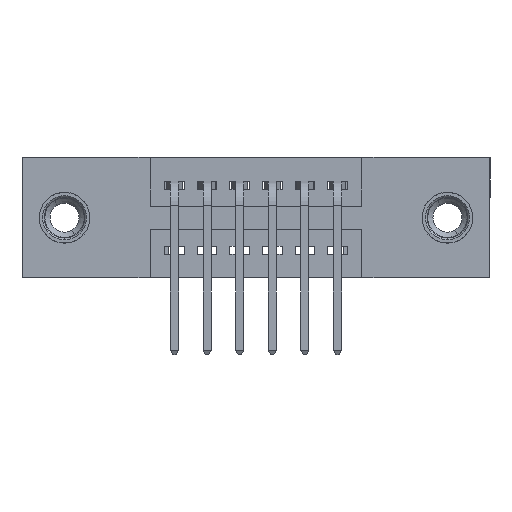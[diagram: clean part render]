
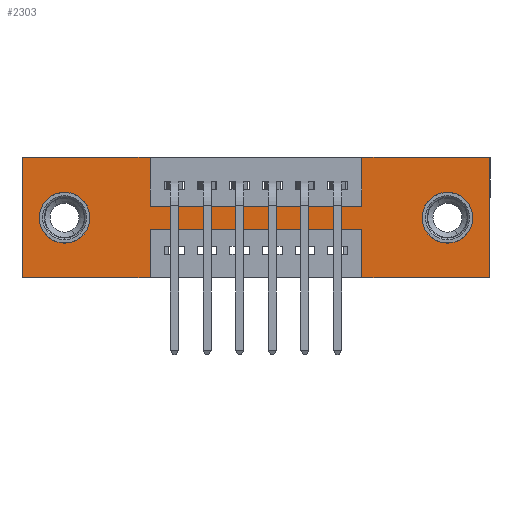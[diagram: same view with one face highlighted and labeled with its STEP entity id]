
A CAD part, front view. The second image highlights one B-rep face of the part: STEP entity #2303.
In plain terms, the highlighted planar face has unit normal (0, -1, 0).
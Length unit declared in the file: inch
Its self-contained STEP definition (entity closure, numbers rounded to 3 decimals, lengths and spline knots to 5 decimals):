
#66 = VERTEX_POINT ( 'NONE', #4925 ) ;
#161 = VECTOR ( 'NONE', #8661, 39.37008 ) ;
#179 = FACE_OUTER_BOUND ( 'NONE', #1727, .T. ) ;
#182 = LINE ( 'NONE', #818, #161 ) ;
#204 = VECTOR ( 'NONE', #8993, 39.37008 ) ;
#225 = FACE_BOUND ( 'NONE', #4309, .T. ) ;
#241 = LINE ( 'NONE', #6955, #1418 ) ;
#306 = FACE_BOUND ( 'NONE', #1010, .T. ) ;
#401 = AXIS2_PLACEMENT_3D ( 'NONE', #2791, #9171, #3927 ) ;
#486 = DIRECTION ( 'NONE',  ( 0., 0., 1. ) ) ;
#660 = VECTOR ( 'NONE', #8094, 39.37008 ) ;
#661 = LINE ( 'NONE', #4678, #204 ) ;
#736 = CIRCLE ( 'NONE', #8279, 0.078 ) ;
#818 = CARTESIAN_POINT ( 'NONE',  ( 0.3925, 0., -0.15 ) ) ;
#853 = LINE ( 'NONE', #2229, #660 ) ;
#1010 = EDGE_LOOP ( 'NONE', ( #11003, #7734 ) ) ;
#1088 = ORIENTED_EDGE ( 'NONE', *, *, #3676, .F. ) ;
#1128 = EDGE_CURVE ( 'NONE', #6700, #6923, #661, .T. ) ;
#1418 = VECTOR ( 'NONE', #8522, 39.37008 ) ;
#1677 = CARTESIAN_POINT ( 'NONE',  ( 0., 0., 0. ) ) ;
#1727 = EDGE_LOOP ( 'NONE', ( #1088, #1945, #2310, #2460, #2490, #3180, #3342, #3688, #4001, #6231, #6503, #6520 ) ) ;
#1875 = VECTOR ( 'NONE', #486, 39.37008 ) ;
#1921 = LINE ( 'NONE', #3873, #1875 ) ;
#1945 = ORIENTED_EDGE ( 'NONE', *, *, #3701, .F. ) ;
#2212 = CARTESIAN_POINT ( 'NONE',  ( 0., 0., -0.37 ) ) ;
#2229 = CARTESIAN_POINT ( 'NONE',  ( 1.435, 0., 0. ) ) ;
#2264 = EDGE_CURVE ( 'NONE', #6988, #7827, #736, .T. ) ;
#2266 = CARTESIAN_POINT ( 'NONE',  ( 1.305, 0., -0.107 ) ) ;
#2303 = ADVANCED_FACE ( 'NONE', ( #225, #306, #179 ), #5395, .T. ) ;
#2310 = ORIENTED_EDGE ( 'NONE', *, *, #3861, .F. ) ;
#2325 = VERTEX_POINT ( 'NONE', #2266 ) ;
#2460 = ORIENTED_EDGE ( 'NONE', *, *, #1128, .F. ) ;
#2490 = ORIENTED_EDGE ( 'NONE', *, *, #11479, .F. ) ;
#2733 = EDGE_CURVE ( 'NONE', #5013, #9312, #11268, .T. ) ;
#2791 = CARTESIAN_POINT ( 'NONE',  ( 0.13, 0., -0.185 ) ) ;
#3017 = CARTESIAN_POINT ( 'NONE',  ( 0.3925, 0., -0.22 ) ) ;
#3030 = LINE ( 'NONE', #8825, #3088 ) ;
#3088 = VECTOR ( 'NONE', #3400, 39.37008 ) ;
#3180 = ORIENTED_EDGE ( 'NONE', *, *, #6342, .F. ) ;
#3212 = EDGE_CURVE ( 'NONE', #2325, #8807, #3395, .T. ) ;
#3314 = EDGE_CURVE ( 'NONE', #8807, #2325, #9994, .T. ) ;
#3335 = DIRECTION ( 'NONE',  ( 0., 0., -1. ) ) ;
#3342 = ORIENTED_EDGE ( 'NONE', *, *, #4095, .F. ) ;
#3395 = CIRCLE ( 'NONE', #4975, 0.078 ) ;
#3400 = DIRECTION ( 'NONE',  ( 0., 0., 1. ) ) ;
#3598 = EDGE_CURVE ( 'NONE', #7827, #6988, #6383, .T. ) ;
#3676 = EDGE_CURVE ( 'NONE', #66, #5013, #6036, .T. ) ;
#3688 = ORIENTED_EDGE ( 'NONE', *, *, #4174, .F. ) ;
#3701 = EDGE_CURVE ( 'NONE', #10763, #66, #5402, .T. ) ;
#3847 = AXIS2_PLACEMENT_3D ( 'NONE', #6434, #11605, #7308 ) ;
#3861 = EDGE_CURVE ( 'NONE', #6923, #10763, #3030, .T. ) ;
#3873 = CARTESIAN_POINT ( 'NONE',  ( 1.0425, 0., 0. ) ) ;
#3927 = DIRECTION ( 'NONE',  ( 0., 0., 1. ) ) ;
#4001 = ORIENTED_EDGE ( 'NONE', *, *, #4557, .F. ) ;
#4095 = EDGE_CURVE ( 'NONE', #4494, #10169, #1921, .T. ) ;
#4174 = EDGE_CURVE ( 'NONE', #8208, #4494, #182, .T. ) ;
#4309 = EDGE_LOOP ( 'NONE', ( #5441, #10403 ) ) ;
#4345 = DIRECTION ( 'NONE',  ( 0., 1., 0. ) ) ;
#4494 = VERTEX_POINT ( 'NONE', #4946 ) ;
#4557 = EDGE_CURVE ( 'NONE', #10348, #8208, #241, .T. ) ;
#4678 = CARTESIAN_POINT ( 'NONE',  ( 0., 0., -0.37 ) ) ;
#4685 = LINE ( 'NONE', #1677, #4804 ) ;
#4780 = VERTEX_POINT ( 'NONE', #10878 ) ;
#4804 = VECTOR ( 'NONE', #7695, 39.37008 ) ;
#4925 = CARTESIAN_POINT ( 'NONE',  ( 0.3925, 0., -0.22 ) ) ;
#4946 = CARTESIAN_POINT ( 'NONE',  ( 1.0425, 0., -0.15 ) ) ;
#4975 = AXIS2_PLACEMENT_3D ( 'NONE', #10816, #6210, #11475 ) ;
#5013 = VERTEX_POINT ( 'NONE', #5685 ) ;
#5263 = CARTESIAN_POINT ( 'NONE',  ( 0., 0., -0.37 ) ) ;
#5272 = VECTOR ( 'NONE', #8614, 39.37008 ) ;
#5344 = DIRECTION ( 'NONE',  ( -1., 0., 0. ) ) ;
#5395 = PLANE ( 'NONE',  #7774 ) ;
#5402 = LINE ( 'NONE', #3017, #5272 ) ;
#5441 = ORIENTED_EDGE ( 'NONE', *, *, #3212, .T. ) ;
#5685 = CARTESIAN_POINT ( 'NONE',  ( 0.3925, 0., -0.37 ) ) ;
#5691 = VECTOR ( 'NONE', #7857, 39.37008 ) ;
#5831 = DIRECTION ( 'NONE',  ( 1., 0., 0. ) ) ;
#5873 = CARTESIAN_POINT ( 'NONE',  ( 1.435, 0., -0.37 ) ) ;
#5980 = VECTOR ( 'NONE', #5831, 39.37008 ) ;
#6036 = LINE ( 'NONE', #11376, #5691 ) ;
#6063 = LINE ( 'NONE', #8385, #5980 ) ;
#6210 = DIRECTION ( 'NONE',  ( 0., 1., 0. ) ) ;
#6231 = ORIENTED_EDGE ( 'NONE', *, *, #8822, .F. ) ;
#6342 = EDGE_CURVE ( 'NONE', #10169, #6797, #11575, .T. ) ;
#6383 = CIRCLE ( 'NONE', #401, 0.078 ) ;
#6434 = CARTESIAN_POINT ( 'NONE',  ( 1.305, 0., -0.185 ) ) ;
#6503 = ORIENTED_EDGE ( 'NONE', *, *, #11208, .F. ) ;
#6520 = ORIENTED_EDGE ( 'NONE', *, *, #2733, .F. ) ;
#6700 = VERTEX_POINT ( 'NONE', #5873 ) ;
#6797 = VERTEX_POINT ( 'NONE', #7771 ) ;
#6923 = VERTEX_POINT ( 'NONE', #7043 ) ;
#6955 = CARTESIAN_POINT ( 'NONE',  ( 0.3925, 0., 0. ) ) ;
#6988 = VERTEX_POINT ( 'NONE', #7974 ) ;
#7043 = CARTESIAN_POINT ( 'NONE',  ( 1.0425, 0., -0.37 ) ) ;
#7308 = DIRECTION ( 'NONE',  ( 0., 0., -1. ) ) ;
#7695 = DIRECTION ( 'NONE',  ( 0., 0., 1. ) ) ;
#7734 = ORIENTED_EDGE ( 'NONE', *, *, #2264, .T. ) ;
#7771 = CARTESIAN_POINT ( 'NONE',  ( 1.435, 0., 0. ) ) ;
#7774 = AXIS2_PLACEMENT_3D ( 'NONE', #2212, #8782, #3335 ) ;
#7827 = VERTEX_POINT ( 'NONE', #8168 ) ;
#7857 = DIRECTION ( 'NONE',  ( 0., 0., -1. ) ) ;
#7861 = CARTESIAN_POINT ( 'NONE',  ( 0.3925, 0., -0.15 ) ) ;
#7974 = CARTESIAN_POINT ( 'NONE',  ( 0.13, 0., -0.263 ) ) ;
#8094 = DIRECTION ( 'NONE',  ( 0., 0., -1. ) ) ;
#8168 = CARTESIAN_POINT ( 'NONE',  ( 0.13, 0., -0.107 ) ) ;
#8182 = CARTESIAN_POINT ( 'NONE',  ( 0., 0., 0. ) ) ;
#8208 = VERTEX_POINT ( 'NONE', #7861 ) ;
#8279 = AXIS2_PLACEMENT_3D ( 'NONE', #9474, #4345, #10235 ) ;
#8385 = CARTESIAN_POINT ( 'NONE',  ( 0., 0., 0. ) ) ;
#8522 = DIRECTION ( 'NONE',  ( 0., 0., -1. ) ) ;
#8580 = CARTESIAN_POINT ( 'NONE',  ( 0.3925, 0., 0. ) ) ;
#8614 = DIRECTION ( 'NONE',  ( -1., 0., 0. ) ) ;
#8661 = DIRECTION ( 'NONE',  ( 1., 0., 0. ) ) ;
#8722 = CARTESIAN_POINT ( 'NONE',  ( 0., 0., -0.37 ) ) ;
#8782 = DIRECTION ( 'NONE',  ( 0., -1., 0. ) ) ;
#8807 = VERTEX_POINT ( 'NONE', #10505 ) ;
#8822 = EDGE_CURVE ( 'NONE', #4780, #10348, #6063, .T. ) ;
#8825 = CARTESIAN_POINT ( 'NONE',  ( 1.0425, 0., -0.37 ) ) ;
#8879 = DIRECTION ( 'NONE',  ( 1., 0., 0. ) ) ;
#8993 = DIRECTION ( 'NONE',  ( -1., 0., 0. ) ) ;
#9171 = DIRECTION ( 'NONE',  ( 0., 1., 0. ) ) ;
#9312 = VERTEX_POINT ( 'NONE', #5263 ) ;
#9474 = CARTESIAN_POINT ( 'NONE',  ( 0.13, 0., -0.185 ) ) ;
#9994 = CIRCLE ( 'NONE', #3847, 0.078 ) ;
#10169 = VERTEX_POINT ( 'NONE', #11535 ) ;
#10235 = DIRECTION ( 'NONE',  ( 0., 0., 1. ) ) ;
#10348 = VERTEX_POINT ( 'NONE', #8580 ) ;
#10403 = ORIENTED_EDGE ( 'NONE', *, *, #3314, .T. ) ;
#10505 = CARTESIAN_POINT ( 'NONE',  ( 1.305, 0., -0.263 ) ) ;
#10689 = CARTESIAN_POINT ( 'NONE',  ( 1.0425, 0., -0.22 ) ) ;
#10763 = VERTEX_POINT ( 'NONE', #10689 ) ;
#10816 = CARTESIAN_POINT ( 'NONE',  ( 1.305, 0., -0.185 ) ) ;
#10878 = CARTESIAN_POINT ( 'NONE',  ( 0., 0., 0. ) ) ;
#11003 = ORIENTED_EDGE ( 'NONE', *, *, #3598, .T. ) ;
#11168 = VECTOR ( 'NONE', #8879, 39.37008 ) ;
#11202 = VECTOR ( 'NONE', #5344, 39.37008 ) ;
#11208 = EDGE_CURVE ( 'NONE', #9312, #4780, #4685, .T. ) ;
#11268 = LINE ( 'NONE', #8722, #11202 ) ;
#11376 = CARTESIAN_POINT ( 'NONE',  ( 0.3925, 0., -0.37 ) ) ;
#11475 = DIRECTION ( 'NONE',  ( 0., 0., -1. ) ) ;
#11479 = EDGE_CURVE ( 'NONE', #6797, #6700, #853, .T. ) ;
#11535 = CARTESIAN_POINT ( 'NONE',  ( 1.0425, 0., 0. ) ) ;
#11575 = LINE ( 'NONE', #8182, #11168 ) ;
#11605 = DIRECTION ( 'NONE',  ( 0., 1., 0. ) ) ;
